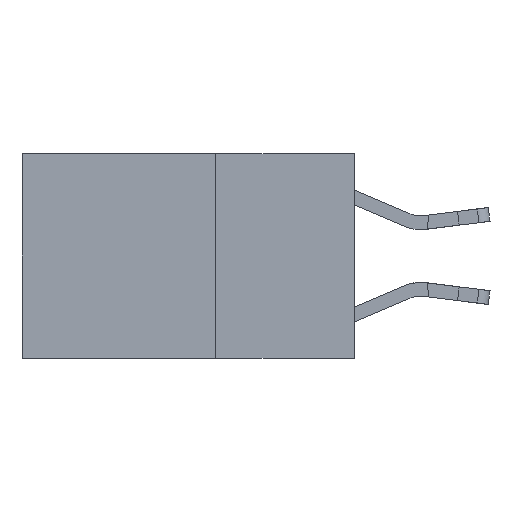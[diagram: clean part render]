
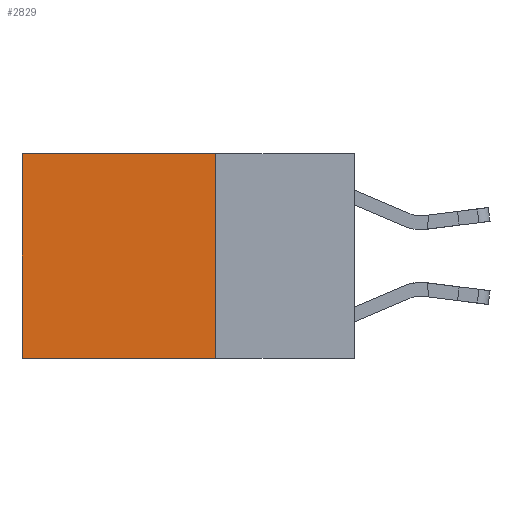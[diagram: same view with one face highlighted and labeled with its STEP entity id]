
A CAD part, left-side view. The second image highlights one B-rep face of the part: STEP entity #2829.
In plain terms, the highlighted planar face has unit normal (-1, 0, 0).
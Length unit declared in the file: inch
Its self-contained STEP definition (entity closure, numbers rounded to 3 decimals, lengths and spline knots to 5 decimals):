
#124 = EDGE_CURVE ( 'NONE', #18815, #14718, #18359, .T. ) ;
#1097 = DIRECTION ( 'NONE',  ( 0., 1., 0. ) ) ;
#1871 = CARTESIAN_POINT ( 'NONE',  ( 0.2625, 0.6, -0.37 ) ) ;
#2801 = VECTOR ( 'NONE', #11168, 39.37008 ) ;
#2829 = ADVANCED_FACE ( 'NONE', ( #4680 ), #11608, .F. ) ;
#2978 = DIRECTION ( 'NONE',  ( 0., 0., -1. ) ) ;
#3879 = VERTEX_POINT ( 'NONE', #1871 ) ;
#4395 = ORIENTED_EDGE ( 'NONE', *, *, #20757, .F. ) ;
#4680 = FACE_OUTER_BOUND ( 'NONE', #6201, .T. ) ;
#4921 = LINE ( 'NONE', #15675, #5298 ) ;
#5247 = CARTESIAN_POINT ( 'NONE',  ( 0.2625, 0.6, 0. ) ) ;
#5298 = VECTOR ( 'NONE', #13767, 39.37008 ) ;
#5919 = LINE ( 'NONE', #11505, #2801 ) ;
#6201 = EDGE_LOOP ( 'NONE', ( #13184, #7157, #4395, #18586 ) ) ;
#6289 = CARTESIAN_POINT ( 'NONE',  ( 0.2625, 0.25, -0.37 ) ) ;
#6375 = VERTEX_POINT ( 'NONE', #6289 ) ;
#7157 = ORIENTED_EDGE ( 'NONE', *, *, #9458, .F. ) ;
#8180 = DIRECTION ( 'NONE',  ( 1., 0., 0. ) ) ;
#9458 = EDGE_CURVE ( 'NONE', #6375, #3879, #5919, .T. ) ;
#11168 = DIRECTION ( 'NONE',  ( 0., 1., 0. ) ) ;
#11505 = CARTESIAN_POINT ( 'NONE',  ( 0.2625, 0.25, -0.37 ) ) ;
#11608 = PLANE ( 'NONE',  #15833 ) ;
#11872 = CARTESIAN_POINT ( 'NONE',  ( 0.2625, 0.6, 0. ) ) ;
#12908 = VECTOR ( 'NONE', #20646, 39.37008 ) ;
#13184 = ORIENTED_EDGE ( 'NONE', *, *, #17721, .T. ) ;
#13396 = VECTOR ( 'NONE', #1097, 39.37008 ) ;
#13767 = DIRECTION ( 'NONE',  ( 0., 0., -1. ) ) ;
#14718 = VERTEX_POINT ( 'NONE', #5247 ) ;
#15675 = CARTESIAN_POINT ( 'NONE',  ( 0.2625, 0.25, 0. ) ) ;
#15833 = AXIS2_PLACEMENT_3D ( 'NONE', #18553, #8180, #2978 ) ;
#16643 = CARTESIAN_POINT ( 'NONE',  ( 0.2625, 0.25, 0. ) ) ;
#17721 = EDGE_CURVE ( 'NONE', #14718, #3879, #20427, .T. ) ;
#18359 = LINE ( 'NONE', #16643, #13396 ) ;
#18553 = CARTESIAN_POINT ( 'NONE',  ( 0.2625, 0.25, 0. ) ) ;
#18586 = ORIENTED_EDGE ( 'NONE', *, *, #124, .T. ) ;
#18815 = VERTEX_POINT ( 'NONE', #20799 ) ;
#20427 = LINE ( 'NONE', #11872, #12908 ) ;
#20646 = DIRECTION ( 'NONE',  ( 0., 0., -1. ) ) ;
#20757 = EDGE_CURVE ( 'NONE', #18815, #6375, #4921, .T. ) ;
#20799 = CARTESIAN_POINT ( 'NONE',  ( 0.2625, 0.25, 0. ) ) ;
